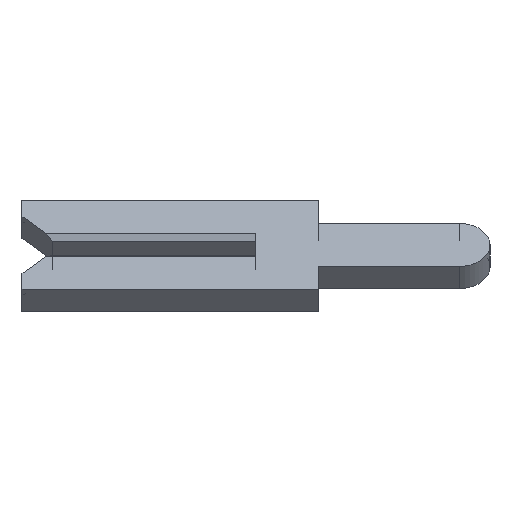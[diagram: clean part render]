
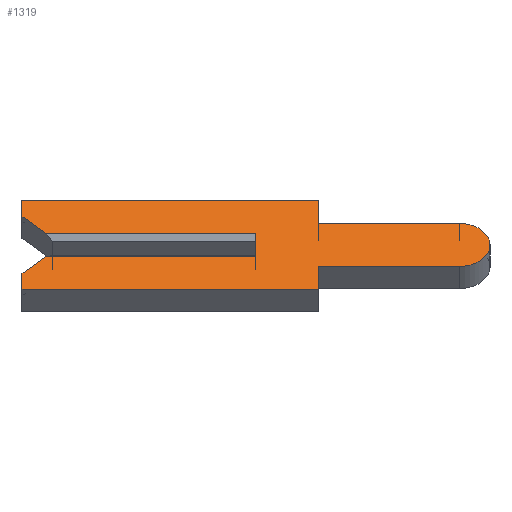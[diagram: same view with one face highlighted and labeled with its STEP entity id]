
A CAD part, left-side view. The second image highlights one B-rep face of the part: STEP entity #1319.
In plain terms, the highlighted face is planar.
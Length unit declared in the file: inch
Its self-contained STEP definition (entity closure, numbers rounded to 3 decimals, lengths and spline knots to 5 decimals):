
#20 = LINE ( 'NONE', #1590, #1355 ) ;
#24 = VECTOR ( 'NONE', #1297, 39.37008 ) ;
#47 = EDGE_CURVE ( 'NONE', #366, #823, #1128, .T. ) ;
#51 = CARTESIAN_POINT ( 'NONE',  ( -0.01, -0.1305, 0.0195 ) ) ;
#56 = CARTESIAN_POINT ( 'NONE',  ( -0.01, 0.1305, 0.0065 ) ) ;
#61 = VERTEX_POINT ( 'NONE', #150 ) ;
#77 = LINE ( 'NONE', #1469, #821 ) ;
#94 = DIRECTION ( 'NONE',  ( 0., 0., 1. ) ) ;
#146 = VECTOR ( 'NONE', #1345, 39.37008 ) ;
#147 = FACE_OUTER_BOUND ( 'NONE', #963, .T. ) ;
#150 = CARTESIAN_POINT ( 'NONE',  ( -0.01, 0.134, 0.01 ) ) ;
#158 = CARTESIAN_POINT ( 'NONE',  ( -0.01, -0.04, -0.04 ) ) ;
#179 = CARTESIAN_POINT ( 'NONE',  ( -0.01, 0., 0.0065 ) ) ;
#187 = VERTEX_POINT ( 'NONE', #51 ) ;
#210 = VERTEX_POINT ( 'NONE', #594 ) ;
#224 = CARTESIAN_POINT ( 'NONE',  ( -0.01, 0.1305, -0.0065 ) ) ;
#240 = DIRECTION ( 'NONE',  ( 0., 0., 1. ) ) ;
#261 = VERTEX_POINT ( 'NONE', #825 ) ;
#269 = EDGE_CURVE ( 'NONE', #591, #549, #1489, .T. ) ;
#277 = CARTESIAN_POINT ( 'NONE',  ( -0.01, -0.04, 0.04 ) ) ;
#285 = DIRECTION ( 'NONE',  ( 0., 0., -1. ) ) ;
#293 = DIRECTION ( 'NONE',  ( 0., 0., -1. ) ) ;
#300 = VECTOR ( 'NONE', #468, 39.37008 ) ;
#322 = VECTOR ( 'NONE', #285, 39.37008 ) ;
#323 = DIRECTION ( 'NONE',  ( 0., 0., -1. ) ) ;
#326 = VERTEX_POINT ( 'NONE', #715 ) ;
#341 = LINE ( 'NONE', #277, #322 ) ;
#366 = VERTEX_POINT ( 'NONE', #1684 ) ;
#369 = CARTESIAN_POINT ( 'NONE',  ( -0.01, 0.15, 0.026 ) ) ;
#406 = ORIENTED_EDGE ( 'NONE', *, *, #809, .F. ) ;
#426 = LINE ( 'NONE', #56, #300 ) ;
#439 = DIRECTION ( 'NONE',  ( 0., 1., 0. ) ) ;
#468 = DIRECTION ( 'NONE',  ( 0., 0.707, 0.707 ) ) ;
#476 = EDGE_CURVE ( 'NONE', #61, #823, #1251, .T. ) ;
#485 = ORIENTED_EDGE ( 'NONE', *, *, #675, .F. ) ;
#549 = VERTEX_POINT ( 'NONE', #1271 ) ;
#555 = DIRECTION ( 'NONE',  ( 1., 0., 0. ) ) ;
#560 = CARTESIAN_POINT ( 'NONE',  ( -0.01, -0.04, -0.0195 ) ) ;
#567 = CARTESIAN_POINT ( 'NONE',  ( -0.01, 0.15, 0.04 ) ) ;
#570 = EDGE_CURVE ( 'NONE', #61, #1086, #426, .T. ) ;
#574 = VERTEX_POINT ( 'NONE', #621 ) ;
#579 = AXIS2_PLACEMENT_3D ( 'NONE', #1702, #1158, #1458 ) ;
#586 = VECTOR ( 'NONE', #993, 39.37008 ) ;
#591 = VERTEX_POINT ( 'NONE', #1045 ) ;
#594 = CARTESIAN_POINT ( 'NONE',  ( -0.01, -0.04, 0.0195 ) ) ;
#621 = CARTESIAN_POINT ( 'NONE',  ( -0.01, -0.1305, -0.0195 ) ) ;
#655 = CARTESIAN_POINT ( 'NONE',  ( -0.01, 0.15, -0.04 ) ) ;
#671 = ORIENTED_EDGE ( 'NONE', *, *, #701, .F. ) ;
#674 = ORIENTED_EDGE ( 'NONE', *, *, #1146, .F. ) ;
#675 = EDGE_CURVE ( 'NONE', #187, #574, #1527, .T. ) ;
#694 = DIRECTION ( 'NONE',  ( 0., -1., 0. ) ) ;
#701 = EDGE_CURVE ( 'NONE', #210, #187, #1081, .T. ) ;
#703 = CARTESIAN_POINT ( 'NONE',  ( -0.01, -0.1305, 0. ) ) ;
#715 = CARTESIAN_POINT ( 'NONE',  ( -0.01, 0.134, -0.01 ) ) ;
#730 = VECTOR ( 'NONE', #439, 39.37008 ) ;
#736 = ORIENTED_EDGE ( 'NONE', *, *, #1456, .F. ) ;
#797 = DIRECTION ( 'NONE',  ( 0., -1., 0. ) ) ;
#809 = EDGE_CURVE ( 'NONE', #1086, #1328, #1524, .T. ) ;
#821 = VECTOR ( 'NONE', #797, 39.37008 ) ;
#823 = VERTEX_POINT ( 'NONE', #1711 ) ;
#825 = CARTESIAN_POINT ( 'NONE',  ( -0.01, -0.04, 0.04 ) ) ;
#830 = ORIENTED_EDGE ( 'NONE', *, *, #873, .F. ) ;
#835 = EDGE_CURVE ( 'NONE', #1064, #1577, #20, .T. ) ;
#847 = ORIENTED_EDGE ( 'NONE', *, *, #1111, .F. ) ;
#873 = EDGE_CURVE ( 'NONE', #1577, #326, #1208, .T. ) ;
#889 = CARTESIAN_POINT ( 'NONE',  ( -0.01, 0.15, 0.01 ) ) ;
#963 = EDGE_LOOP ( 'NONE', ( #1108, #1452, #984, #830, #1153, #847, #1048, #1132, #485, #671, #674, #736, #406, #1514 ) ) ;
#984 = ORIENTED_EDGE ( 'NONE', *, *, #1120, .F. ) ;
#993 = DIRECTION ( 'NONE',  ( 0., -1., 0. ) ) ;
#996 = VECTOR ( 'NONE', #323, 39.37008 ) ;
#1010 = AXIS2_PLACEMENT_3D ( 'NONE', #703, #555, #293 ) ;
#1045 = CARTESIAN_POINT ( 'NONE',  ( -0.01, -0.04, -0.0195 ) ) ;
#1048 = ORIENTED_EDGE ( 'NONE', *, *, #269, .F. ) ;
#1064 = VERTEX_POINT ( 'NONE', #655 ) ;
#1066 = CARTESIAN_POINT ( 'NONE',  ( -0.01, 0.15, 0.026 ) ) ;
#1081 = LINE ( 'NONE', #1583, #24 ) ;
#1086 = VERTEX_POINT ( 'NONE', #1066 ) ;
#1090 = VECTOR ( 'NONE', #694, 39.37008 ) ;
#1108 = ORIENTED_EDGE ( 'NONE', *, *, #476, .T. ) ;
#1111 = EDGE_CURVE ( 'NONE', #549, #1064, #1644, .T. ) ;
#1120 = EDGE_CURVE ( 'NONE', #326, #366, #77, .T. ) ;
#1128 = LINE ( 'NONE', #179, #146 ) ;
#1132 = ORIENTED_EDGE ( 'NONE', *, *, #1243, .F. ) ;
#1146 = EDGE_CURVE ( 'NONE', #261, #210, #341, .T. ) ;
#1153 = ORIENTED_EDGE ( 'NONE', *, *, #835, .F. ) ;
#1158 = DIRECTION ( 'NONE',  ( 1., 0., 0. ) ) ;
#1188 = VECTOR ( 'NONE', #240, 39.37008 ) ;
#1208 = LINE ( 'NONE', #224, #1546 ) ;
#1212 = VECTOR ( 'NONE', #1604, 39.37008 ) ;
#1243 = EDGE_CURVE ( 'NONE', #574, #591, #1363, .T. ) ;
#1251 = LINE ( 'NONE', #889, #586 ) ;
#1255 = CARTESIAN_POINT ( 'NONE',  ( -0.01, 0.15, -0.026 ) ) ;
#1271 = CARTESIAN_POINT ( 'NONE',  ( -0.01, -0.04, -0.04 ) ) ;
#1297 = DIRECTION ( 'NONE',  ( 0., -1., 0. ) ) ;
#1319 = ADVANCED_FACE ( 'NONE', ( #147 ), #1358, .F. ) ;
#1324 = CARTESIAN_POINT ( 'NONE',  ( -0.01, 0.15, -0.04 ) ) ;
#1328 = VERTEX_POINT ( 'NONE', #567 ) ;
#1345 = DIRECTION ( 'NONE',  ( 0., 0., 1. ) ) ;
#1355 = VECTOR ( 'NONE', #94, 39.37008 ) ;
#1358 = PLANE ( 'NONE',  #1010 ) ;
#1363 = LINE ( 'NONE', #560, #730 ) ;
#1374 = CARTESIAN_POINT ( 'NONE',  ( -0.01, 0.15, 0.04 ) ) ;
#1452 = ORIENTED_EDGE ( 'NONE', *, *, #47, .F. ) ;
#1456 = EDGE_CURVE ( 'NONE', #1328, #261, #1580, .T. ) ;
#1458 = DIRECTION ( 'NONE',  ( 0., 0., -1. ) ) ;
#1469 = CARTESIAN_POINT ( 'NONE',  ( -0.01, -0.1305, -0.01 ) ) ;
#1476 = DIRECTION ( 'NONE',  ( 0., -0.707, 0.707 ) ) ;
#1489 = LINE ( 'NONE', #158, #996 ) ;
#1514 = ORIENTED_EDGE ( 'NONE', *, *, #570, .F. ) ;
#1524 = LINE ( 'NONE', #369, #1188 ) ;
#1527 = CIRCLE ( 'NONE', #579, 0.0195 ) ;
#1546 = VECTOR ( 'NONE', #1476, 39.37008 ) ;
#1577 = VERTEX_POINT ( 'NONE', #1255 ) ;
#1580 = LINE ( 'NONE', #1374, #1090 ) ;
#1583 = CARTESIAN_POINT ( 'NONE',  ( -0.01, -0.04, 0.0195 ) ) ;
#1590 = CARTESIAN_POINT ( 'NONE',  ( -0.01, 0.15, -0.026 ) ) ;
#1604 = DIRECTION ( 'NONE',  ( 0., 1., 0. ) ) ;
#1644 = LINE ( 'NONE', #1324, #1212 ) ;
#1684 = CARTESIAN_POINT ( 'NONE',  ( -0.01, 0., -0.01 ) ) ;
#1702 = CARTESIAN_POINT ( 'NONE',  ( -0.01, -0.1305, 0. ) ) ;
#1711 = CARTESIAN_POINT ( 'NONE',  ( -0.01, 0., 0.01 ) ) ;
